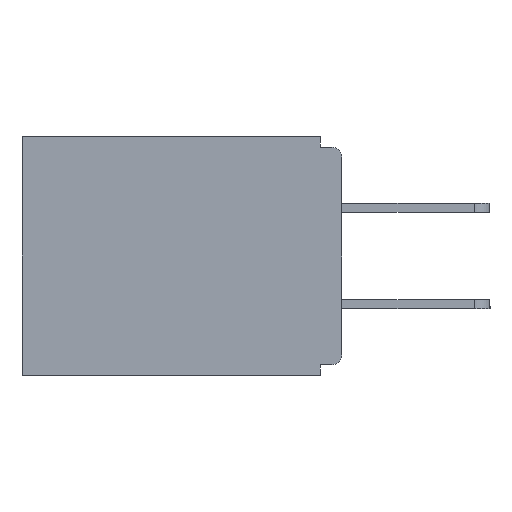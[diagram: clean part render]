
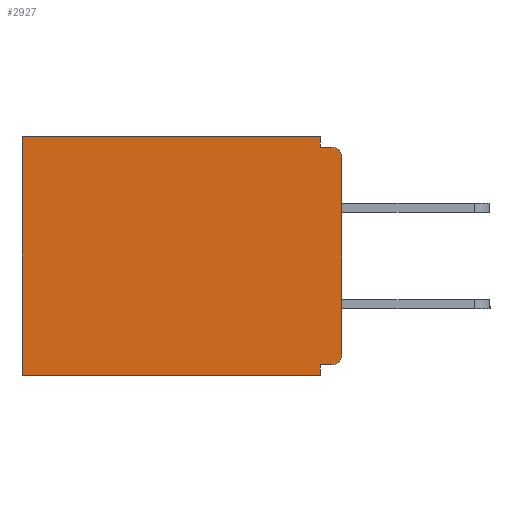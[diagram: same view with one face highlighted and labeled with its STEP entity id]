
A CAD part, left-side view. The second image highlights one B-rep face of the part: STEP entity #2927.
In plain terms, the highlighted planar face has unit normal (-1, 0, 0).
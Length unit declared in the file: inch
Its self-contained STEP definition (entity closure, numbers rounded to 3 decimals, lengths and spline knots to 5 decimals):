
#61 = LINE ( 'NONE', #411, #9732 ) ;
#411 = CARTESIAN_POINT ( 'NONE',  ( 0.298, 0., 0. ) ) ;
#413 = CARTESIAN_POINT ( 'NONE',  ( 0.298, 0.031, -0.328 ) ) ;
#541 = CARTESIAN_POINT ( 'NONE',  ( 0.298, 0., 0. ) ) ;
#718 = LINE ( 'NONE', #7972, #6995 ) ;
#820 = EDGE_LOOP ( 'NONE', ( #9333, #8937, #7477, #3054, #10077, #9153, #7409, #5474, #10453, #6466 ) ) ;
#1180 = CARTESIAN_POINT ( 'NONE',  ( 0.298, 0.015, -0.313 ) ) ;
#1411 = LINE ( 'NONE', #7053, #1577 ) ;
#1510 = EDGE_CURVE ( 'NONE', #13132, #6945, #3398, .T. ) ;
#1577 = VECTOR ( 'NONE', #9101, 39.37008 ) ;
#1605 = DIRECTION ( 'NONE',  ( 0., 1., 0. ) ) ;
#1628 = VERTEX_POINT ( 'NONE', #2391 ) ;
#2009 = DIRECTION ( 'NONE',  ( 0., -1., 0. ) ) ;
#2030 = DIRECTION ( 'NONE',  ( -1., 0., 0. ) ) ;
#2061 = DIRECTION ( 'NONE',  ( -1., 0., 0. ) ) ;
#2391 = CARTESIAN_POINT ( 'NONE',  ( 0.298, 0., -0.313 ) ) ;
#2398 = LINE ( 'NONE', #5497, #9204 ) ;
#2408 = VERTEX_POINT ( 'NONE', #10770 ) ;
#2510 = EDGE_CURVE ( 'NONE', #2408, #4528, #4999, .T. ) ;
#2927 = ADVANCED_FACE ( 'NONE', ( #4024 ), #7713, .F. ) ;
#2937 = DIRECTION ( 'NONE',  ( 0., 0., -1. ) ) ;
#3000 = CARTESIAN_POINT ( 'NONE',  ( 0.298, 0., -0.015 ) ) ;
#3054 = ORIENTED_EDGE ( 'NONE', *, *, #6513, .T. ) ;
#3121 = VERTEX_POINT ( 'NONE', #5360 ) ;
#3334 = VERTEX_POINT ( 'NONE', #10911 ) ;
#3398 = LINE ( 'NONE', #11485, #9884 ) ;
#4024 = FACE_OUTER_BOUND ( 'NONE', #820, .T. ) ;
#4101 = CIRCLE ( 'NONE', #13152, 0.015 ) ;
#4236 = AXIS2_PLACEMENT_3D ( 'NONE', #11401, #2030, #8140 ) ;
#4269 = EDGE_CURVE ( 'NONE', #3121, #4528, #4451, .T. ) ;
#4451 = CIRCLE ( 'NONE', #4236, 0.015 ) ;
#4528 = VERTEX_POINT ( 'NONE', #4619 ) ;
#4619 = CARTESIAN_POINT ( 'NONE',  ( 0.298, 0.015, -0.015 ) ) ;
#4754 = DIRECTION ( 'NONE',  ( 1., 0., 0. ) ) ;
#4999 = LINE ( 'NONE', #3000, #9055 ) ;
#5299 = DIRECTION ( 'NONE',  ( 0., 1., 0. ) ) ;
#5327 = EDGE_CURVE ( 'NONE', #13132, #1628, #4101, .T. ) ;
#5360 = CARTESIAN_POINT ( 'NONE',  ( 0.298, 0., -0.03 ) ) ;
#5474 = ORIENTED_EDGE ( 'NONE', *, *, #1510, .F. ) ;
#5497 = CARTESIAN_POINT ( 'NONE',  ( 0.298, 0.031, -0.343 ) ) ;
#5624 = CARTESIAN_POINT ( 'NONE',  ( 0.298, 0.46, -0.343 ) ) ;
#5703 = VERTEX_POINT ( 'NONE', #5624 ) ;
#6317 = CARTESIAN_POINT ( 'NONE',  ( 0.298, 0.015, -0.328 ) ) ;
#6466 = ORIENTED_EDGE ( 'NONE', *, *, #12807, .F. ) ;
#6513 = EDGE_CURVE ( 'NONE', #3334, #7457, #8212, .T. ) ;
#6670 = EDGE_CURVE ( 'NONE', #9360, #5703, #1411, .T. ) ;
#6945 = VERTEX_POINT ( 'NONE', #413 ) ;
#6995 = VECTOR ( 'NONE', #2937, 39.37008 ) ;
#7053 = CARTESIAN_POINT ( 'NONE',  ( 0.298, 0., -0.343 ) ) ;
#7409 = ORIENTED_EDGE ( 'NONE', *, *, #9697, .F. ) ;
#7424 = DIRECTION ( 'NONE',  ( 0., 0., -1. ) ) ;
#7457 = VERTEX_POINT ( 'NONE', #12404 ) ;
#7477 = ORIENTED_EDGE ( 'NONE', *, *, #12294, .F. ) ;
#7538 = DIRECTION ( 'NONE',  ( 0., 0., -1. ) ) ;
#7604 = EDGE_CURVE ( 'NONE', #7457, #5703, #12849, .T. ) ;
#7713 = PLANE ( 'NONE',  #12262 ) ;
#7736 = VECTOR ( 'NONE', #1605, 39.37008 ) ;
#7972 = CARTESIAN_POINT ( 'NONE',  ( 0.298, 0.031, -0.343 ) ) ;
#8075 = DIRECTION ( 'NONE',  ( 0., 0., -1. ) ) ;
#8140 = DIRECTION ( 'NONE',  ( 0., 0., -1. ) ) ;
#8212 = LINE ( 'NONE', #10043, #7736 ) ;
#8849 = DIRECTION ( 'NONE',  ( 0., 0., -1. ) ) ;
#8937 = ORIENTED_EDGE ( 'NONE', *, *, #2510, .F. ) ;
#9055 = VECTOR ( 'NONE', #2009, 39.37008 ) ;
#9101 = DIRECTION ( 'NONE',  ( 0., 1., 0. ) ) ;
#9153 = ORIENTED_EDGE ( 'NONE', *, *, #6670, .F. ) ;
#9204 = VECTOR ( 'NONE', #7424, 39.37008 ) ;
#9333 = ORIENTED_EDGE ( 'NONE', *, *, #4269, .T. ) ;
#9360 = VERTEX_POINT ( 'NONE', #12877 ) ;
#9697 = EDGE_CURVE ( 'NONE', #6945, #9360, #718, .T. ) ;
#9732 = VECTOR ( 'NONE', #7538, 39.37008 ) ;
#9884 = VECTOR ( 'NONE', #5299, 39.37008 ) ;
#10043 = CARTESIAN_POINT ( 'NONE',  ( 0.298, 0., 0. ) ) ;
#10077 = ORIENTED_EDGE ( 'NONE', *, *, #7604, .T. ) ;
#10453 = ORIENTED_EDGE ( 'NONE', *, *, #5327, .T. ) ;
#10770 = CARTESIAN_POINT ( 'NONE',  ( 0.298, 0.031, -0.015 ) ) ;
#10911 = CARTESIAN_POINT ( 'NONE',  ( 0.298, 0.031, 0. ) ) ;
#11146 = CARTESIAN_POINT ( 'NONE',  ( 0.298, 0.46, 0. ) ) ;
#11401 = CARTESIAN_POINT ( 'NONE',  ( 0.298, 0.015, -0.03 ) ) ;
#11485 = CARTESIAN_POINT ( 'NONE',  ( 0.298, 0., -0.328 ) ) ;
#12212 = VECTOR ( 'NONE', #8075, 39.37008 ) ;
#12262 = AXIS2_PLACEMENT_3D ( 'NONE', #541, #4754, #8849 ) ;
#12294 = EDGE_CURVE ( 'NONE', #3334, #2408, #2398, .T. ) ;
#12404 = CARTESIAN_POINT ( 'NONE',  ( 0.298, 0.46, 0. ) ) ;
#12487 = DIRECTION ( 'NONE',  ( 0., 0., -1. ) ) ;
#12807 = EDGE_CURVE ( 'NONE', #3121, #1628, #61, .T. ) ;
#12849 = LINE ( 'NONE', #11146, #12212 ) ;
#12877 = CARTESIAN_POINT ( 'NONE',  ( 0.298, 0.031, -0.343 ) ) ;
#13132 = VERTEX_POINT ( 'NONE', #6317 ) ;
#13152 = AXIS2_PLACEMENT_3D ( 'NONE', #1180, #2061, #12487 ) ;
